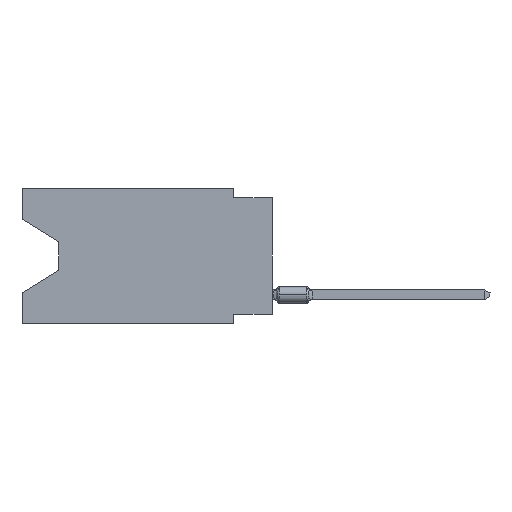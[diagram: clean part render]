
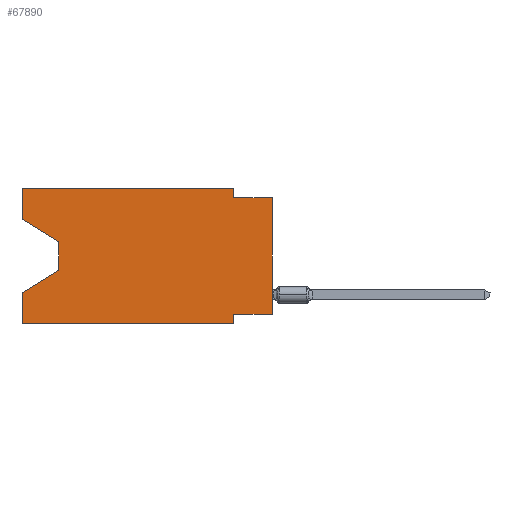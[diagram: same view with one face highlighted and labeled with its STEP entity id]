
A CAD part, left-side view. The second image highlights one B-rep face of the part: STEP entity #67890.
In plain terms, the highlighted planar face has unit normal (-1, 0, 0).
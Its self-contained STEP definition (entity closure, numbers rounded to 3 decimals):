
#1484 = VECTOR ( 'NONE', #62826, 1000. ) ;
#3799 = LINE ( 'NONE', #43861, #19334 ) ;
#4991 = EDGE_CURVE ( 'NONE', #65949, #21049, #52889, .T. ) ;
#6102 = EDGE_CURVE ( 'NONE', #61143, #10392, #73236, .T. ) ;
#6168 = DIRECTION ( 'NONE',  ( 0., -1., 0. ) ) ;
#7747 = CARTESIAN_POINT ( 'NONE',  ( 0., 13.97, -3.505 ) ) ;
#7989 = VECTOR ( 'NONE', #67074, 1000. ) ;
#8739 = EDGE_CURVE ( 'NONE', #19019, #70333, #3799, .T. ) ;
#9081 = CARTESIAN_POINT ( 'NONE',  ( 0., 0., -0.635 ) ) ;
#9164 = PLANE ( 'NONE',  #23688 ) ;
#9233 = EDGE_CURVE ( 'NONE', #43526, #31683, #28075, .T. ) ;
#9476 = LINE ( 'NONE', #14073, #7989 ) ;
#9828 = VERTEX_POINT ( 'NONE', #24565 ) ;
#10065 = CARTESIAN_POINT ( 'NONE',  ( 0., 16.383, -2.038 ) ) ;
#10291 = VERTEX_POINT ( 'NONE', #9081 ) ;
#10392 = VERTEX_POINT ( 'NONE', #74246 ) ;
#14073 = CARTESIAN_POINT ( 'NONE',  ( 0., 16.383, -8.89 ) ) ;
#14699 = CARTESIAN_POINT ( 'NONE',  ( 0., 2.54, 0. ) ) ;
#14820 = ORIENTED_EDGE ( 'NONE', *, *, #6102, .F. ) ;
#15423 = EDGE_CURVE ( 'NONE', #9828, #10291, #33863, .T. ) ;
#16307 = CARTESIAN_POINT ( 'NONE',  ( 0., 13.97, -5.385 ) ) ;
#17433 = CARTESIAN_POINT ( 'NONE',  ( 0., 2.54, -8.89 ) ) ;
#18291 = ORIENTED_EDGE ( 'NONE', *, *, #45669, .F. ) ;
#19019 = VERTEX_POINT ( 'NONE', #70487 ) ;
#19334 = VECTOR ( 'NONE', #32771, 1000. ) ;
#19773 = EDGE_CURVE ( 'NONE', #70333, #61241, #53147, .T. ) ;
#21049 = VERTEX_POINT ( 'NONE', #7747 ) ;
#21092 = ORIENTED_EDGE ( 'NONE', *, *, #35188, .T. ) ;
#23688 = AXIS2_PLACEMENT_3D ( 'NONE', #61777, #44974, #68619 ) ;
#24565 = CARTESIAN_POINT ( 'NONE',  ( 0., 0., -8.255 ) ) ;
#25793 = EDGE_CURVE ( 'NONE', #61143, #31683, #9476, .T. ) ;
#26064 = EDGE_CURVE ( 'NONE', #21049, #54961, #64358, .T. ) ;
#27518 = VECTOR ( 'NONE', #51464, 1000. ) ;
#27796 = CARTESIAN_POINT ( 'NONE',  ( 0., 16.383, -8.89 ) ) ;
#28075 = LINE ( 'NONE', #17433, #63170 ) ;
#28504 = EDGE_LOOP ( 'NONE', ( #45185, #54600, #21092, #14820, #56533, #65838, #34522, #69711, #39791, #35775, #66139, #18291 ) ) ;
#28536 = VECTOR ( 'NONE', #55968, 1000. ) ;
#31683 = VERTEX_POINT ( 'NONE', #39677 ) ;
#31768 = CARTESIAN_POINT ( 'NONE',  ( 0., 2.54, -8.255 ) ) ;
#31952 = CARTESIAN_POINT ( 'NONE',  ( 0., 13.97, -5.385 ) ) ;
#32771 = DIRECTION ( 'NONE',  ( 0., -1., 0. ) ) ;
#33863 = LINE ( 'NONE', #57132, #40604 ) ;
#34522 = ORIENTED_EDGE ( 'NONE', *, *, #68551, .F. ) ;
#35136 = LINE ( 'NONE', #47352, #55712 ) ;
#35188 = EDGE_CURVE ( 'NONE', #54961, #10392, #45292, .T. ) ;
#35775 = ORIENTED_EDGE ( 'NONE', *, *, #19773, .F. ) ;
#36100 = CARTESIAN_POINT ( 'NONE',  ( 0., 0., -8.255 ) ) ;
#36836 = CARTESIAN_POINT ( 'NONE',  ( 0., 16.383, -2.038 ) ) ;
#39677 = CARTESIAN_POINT ( 'NONE',  ( 0., 2.54, -8.89 ) ) ;
#39791 = ORIENTED_EDGE ( 'NONE', *, *, #49907, .F. ) ;
#40377 = VECTOR ( 'NONE', #41705, 1000. ) ;
#40604 = VECTOR ( 'NONE', #51423, 1000. ) ;
#41068 = DIRECTION ( 'NONE',  ( 0., 0., -1. ) ) ;
#41705 = DIRECTION ( 'NONE',  ( 0., 0., -1. ) ) ;
#42232 = VECTOR ( 'NONE', #60109, 1000. ) ;
#43526 = VERTEX_POINT ( 'NONE', #31768 ) ;
#43861 = CARTESIAN_POINT ( 'NONE',  ( 0., 16.383, 0. ) ) ;
#44974 = DIRECTION ( 'NONE',  ( 1., 0., 0. ) ) ;
#45185 = ORIENTED_EDGE ( 'NONE', *, *, #4991, .T. ) ;
#45292 = LINE ( 'NONE', #16307, #1484 ) ;
#45352 = FACE_OUTER_BOUND ( 'NONE', #28504, .T. ) ;
#45669 = EDGE_CURVE ( 'NONE', #65949, #19019, #50254, .T. ) ;
#47169 = DIRECTION ( 'NONE',  ( 0., -0.855, -0.519 ) ) ;
#47352 = CARTESIAN_POINT ( 'NONE',  ( 0., 0., -0.635 ) ) ;
#47927 = LINE ( 'NONE', #36100, #42232 ) ;
#49907 = EDGE_CURVE ( 'NONE', #61241, #10291, #35136, .T. ) ;
#50254 = LINE ( 'NONE', #62798, #28536 ) ;
#50453 = VECTOR ( 'NONE', #47169, 1000. ) ;
#51423 = DIRECTION ( 'NONE',  ( 0., 0., 1. ) ) ;
#51464 = DIRECTION ( 'NONE',  ( 0., 0., 1. ) ) ;
#52889 = LINE ( 'NONE', #36836, #50453 ) ;
#52922 = CARTESIAN_POINT ( 'NONE',  ( 0., 13.97, -3.505 ) ) ;
#53147 = LINE ( 'NONE', #59980, #40377 ) ;
#54600 = ORIENTED_EDGE ( 'NONE', *, *, #26064, .T. ) ;
#54961 = VERTEX_POINT ( 'NONE', #31952 ) ;
#55712 = VECTOR ( 'NONE', #6168, 1000. ) ;
#55968 = DIRECTION ( 'NONE',  ( 0., 0., 1. ) ) ;
#56533 = ORIENTED_EDGE ( 'NONE', *, *, #25793, .T. ) ;
#57132 = CARTESIAN_POINT ( 'NONE',  ( 0., 0., 0. ) ) ;
#59003 = DIRECTION ( 'NONE',  ( 0., 0., -1. ) ) ;
#59980 = CARTESIAN_POINT ( 'NONE',  ( 0., 2.54, 0. ) ) ;
#60109 = DIRECTION ( 'NONE',  ( 0., 1., 0. ) ) ;
#61143 = VERTEX_POINT ( 'NONE', #27796 ) ;
#61241 = VERTEX_POINT ( 'NONE', #71273 ) ;
#61777 = CARTESIAN_POINT ( 'NONE',  ( 0., 16.383, 0. ) ) ;
#62798 = CARTESIAN_POINT ( 'NONE',  ( 0., 16.383, 0. ) ) ;
#62826 = DIRECTION ( 'NONE',  ( 0., 0.855, -0.519 ) ) ;
#63170 = VECTOR ( 'NONE', #41068, 1000. ) ;
#64358 = LINE ( 'NONE', #52922, #71372 ) ;
#65838 = ORIENTED_EDGE ( 'NONE', *, *, #9233, .F. ) ;
#65949 = VERTEX_POINT ( 'NONE', #10065 ) ;
#66139 = ORIENTED_EDGE ( 'NONE', *, *, #8739, .F. ) ;
#67074 = DIRECTION ( 'NONE',  ( 0., -1., 0. ) ) ;
#67878 = CARTESIAN_POINT ( 'NONE',  ( 0., 16.383, 0. ) ) ;
#67890 = ADVANCED_FACE ( 'NONE', ( #45352 ), #9164, .F. ) ;
#68551 = EDGE_CURVE ( 'NONE', #9828, #43526, #47927, .T. ) ;
#68619 = DIRECTION ( 'NONE',  ( 0., 0., -1. ) ) ;
#69711 = ORIENTED_EDGE ( 'NONE', *, *, #15423, .T. ) ;
#70333 = VERTEX_POINT ( 'NONE', #14699 ) ;
#70487 = CARTESIAN_POINT ( 'NONE',  ( 0., 16.383, 0. ) ) ;
#71273 = CARTESIAN_POINT ( 'NONE',  ( 0., 2.54, -0.635 ) ) ;
#71372 = VECTOR ( 'NONE', #59003, 1000. ) ;
#73236 = LINE ( 'NONE', #67878, #27518 ) ;
#74246 = CARTESIAN_POINT ( 'NONE',  ( 0., 16.383, -6.852 ) ) ;
